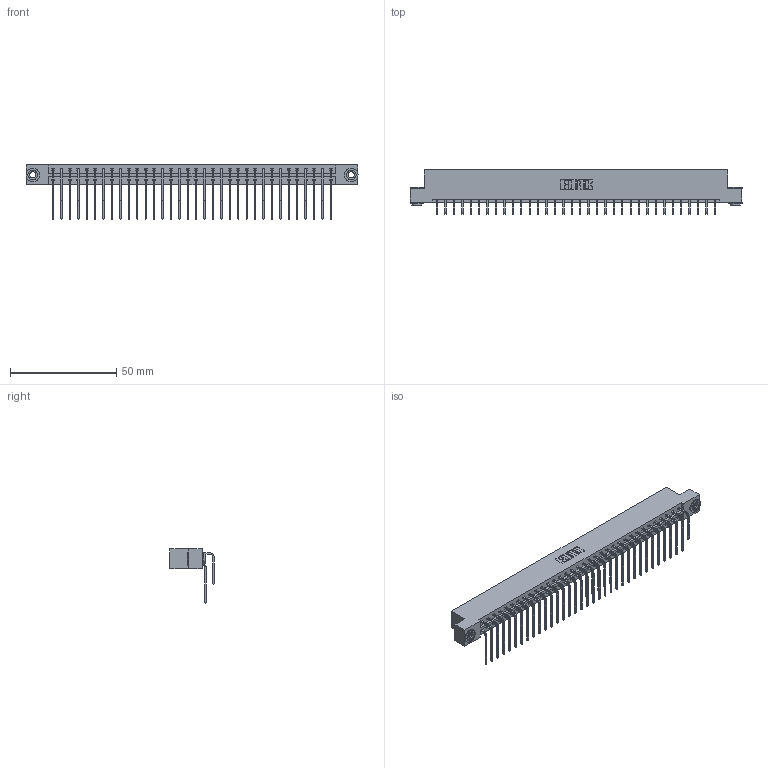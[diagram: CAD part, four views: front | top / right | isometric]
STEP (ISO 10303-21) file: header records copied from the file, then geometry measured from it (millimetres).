
FILE_DESCRIPTION (( 'STEP AP203' ), '1' );
FILE_NAME ('833-068-559-203.STEP', '2020-06-05T11:26:41', ( '' ), ( '' ), 'SwSTEP 2.0', 'SolidWorks 2020', '' );
FILE_SCHEMA (( 'CONFIG_CONTROL_DESIGN' ));
Length unit declared in the file: inch
Products named in the file (5): 833-068-559-203; 345-250-002_345-250-002-102; 345-292-001_559 Tail - 2; 833 Part_Flush - .156 Dia - TH; 345-292-001_558 559 Tail - 1
Assembly tree (71 placements, depth 2):
  833-068-559-203
    833 Part_Flush - .156 Dia - TH
    345-292-001_558 559 Tail - 1  x34
    345-292-001_559 Tail - 2  x34
    345-250-002_345-250-002-102  x2
Bounding box: 156.26 x 20.9 x 25.53 mm (x, y, z)
Volume: 16290.2 mm3; surface area: 21347.9 mm2
Topology: 71 solids, 71 shells, 3824 faces, 11335 edges, 7462 vertices
Faces by surface type: plane 2664, cylinder 1152, cone 8
Entity records: 25342 total; most frequent: CARTESIAN_POINT 4236, ORIENTED_EDGE 4114, DIRECTION 3647, EDGE_CURVE 2057, LINE 1865, VECTOR 1865, VERTEX_POINT 1366, AXIS2_PLACEMENT_3D 891
